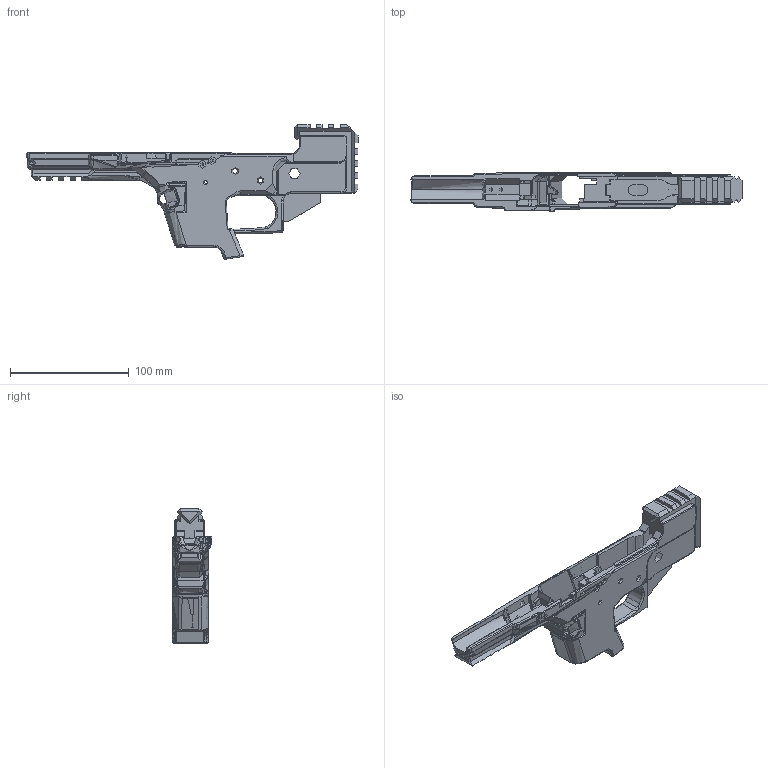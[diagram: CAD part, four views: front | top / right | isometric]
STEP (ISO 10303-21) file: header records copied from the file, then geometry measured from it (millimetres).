
FILE_DESCRIPTION (( 'STEP AP214' ), '1' );
FILE_NAME ('3089 Frame RaR.STEP', '2022-08-26T00:50:24', ( '' ), ( '' ), 'SwSTEP 2.0', 'SolidWorks 2020', '' );
FILE_SCHEMA (( 'AUTOMOTIVE_DESIGN' ));
Length unit declared in the file: millimetre
Products named in the file (1): 3089 Frame RaR
Bounding box: 279.81 x 32.88 x 113.49 mm (x, y, z)
Topology: 0 solids, 3 shells, 1537 faces, 4232 edges, 2667 vertices
Faces by surface type: plane 537, bspline 492, cylinder 379, torus 76, cone 45, sphere 8
Entity records: 75745 total; most frequent: CARTESIAN_POINT 42480, ORIENTED_EDGE 8406, DIRECTION 4930, EDGE_CURVE 4203, VERTEX_POINT 2662, B_SPLINE_CURVE_WITH_KNOTS 1746, AXIS2_PLACEMENT_3D 1712, EDGE_LOOP 1577
